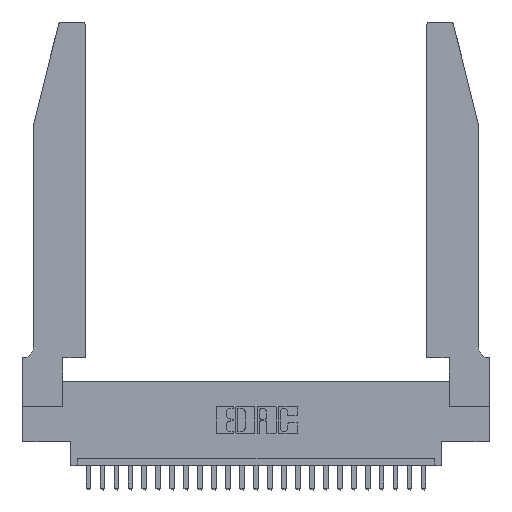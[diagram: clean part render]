
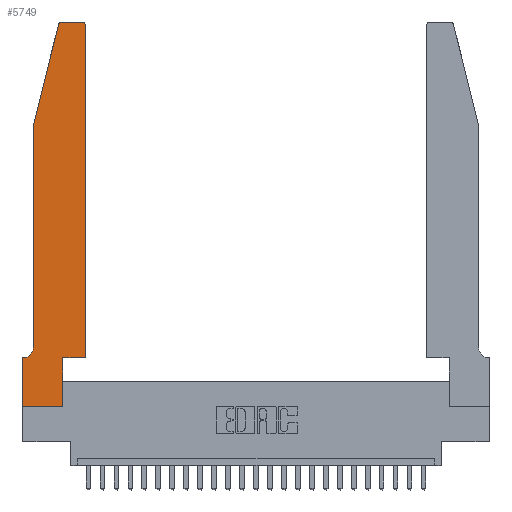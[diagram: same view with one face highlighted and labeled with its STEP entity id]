
A CAD part, top view. The second image highlights one B-rep face of the part: STEP entity #5749.
In plain terms, the highlighted planar face has unit normal (0, 0, 1).
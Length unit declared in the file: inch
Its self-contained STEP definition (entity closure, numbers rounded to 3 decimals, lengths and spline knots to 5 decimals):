
#238 = ORIENTED_EDGE ( 'NONE', *, *, #6319, .T. ) ;
#380 = DIRECTION ( 'NONE',  ( 1., 0., 0. ) ) ;
#554 = AXIS2_PLACEMENT_3D ( 'NONE', #16394, #8370, #4819 ) ;
#911 = VERTEX_POINT ( 'NONE', #15841 ) ;
#964 = DIRECTION ( 'NONE',  ( 1., 0., 0. ) ) ;
#1431 = EDGE_CURVE ( 'NONE', #16127, #13014, #11817, .T. ) ;
#2209 = LINE ( 'NONE', #9297, #5971 ) ;
#2292 = LINE ( 'NONE', #18422, #3536 ) ;
#2298 = PLANE ( 'NONE',  #554 ) ;
#2306 = CARTESIAN_POINT ( 'NONE',  ( 0.25487, 2.72718, 0.37 ) ) ;
#2475 = LINE ( 'NONE', #12851, #16607 ) ;
#2971 = ORIENTED_EDGE ( 'NONE', *, *, #1431, .T. ) ;
#3141 = ORIENTED_EDGE ( 'NONE', *, *, #25940, .T. ) ;
#3298 = EDGE_CURVE ( 'NONE', #3597, #13988, #22091, .T. ) ;
#3417 = CARTESIAN_POINT ( 'NONE',  ( 0.284, 2.75, 0.37 ) ) ;
#3482 = VECTOR ( 'NONE', #380, 39.37008 ) ;
#3536 = VECTOR ( 'NONE', #10362, 39.37008 ) ;
#3597 = VERTEX_POINT ( 'NONE', #12074 ) ;
#3706 = VERTEX_POINT ( 'NONE', #9615 ) ;
#3900 = ORIENTED_EDGE ( 'NONE', *, *, #3298, .T. ) ;
#3927 = VECTOR ( 'NONE', #9488, 39.37008 ) ;
#4383 = CARTESIAN_POINT ( 'NONE',  ( 0.4505, 0.35, 0.37 ) ) ;
#4387 = AXIS2_PLACEMENT_3D ( 'NONE', #4671, #24674, #16696 ) ;
#4437 = VECTOR ( 'NONE', #12284, 39.37008 ) ;
#4560 = CARTESIAN_POINT ( 'NONE',  ( 0.4205, 2.75, 0.37 ) ) ;
#4671 = CARTESIAN_POINT ( 'NONE',  ( 0.284, 2.72, 0.37 ) ) ;
#4819 = DIRECTION ( 'NONE',  ( 1., 0., 0. ) ) ;
#5542 = ORIENTED_EDGE ( 'NONE', *, *, #9561, .T. ) ;
#5701 = CARTESIAN_POINT ( 'NONE',  ( 0.4205, 2.72, 0.37 ) ) ;
#5749 = ADVANCED_FACE ( 'NONE', ( #19429 ), #2298, .T. ) ;
#5970 = DIRECTION ( 'NONE',  ( 0., 0., -1. ) ) ;
#5971 = VECTOR ( 'NONE', #22456, 39.37008 ) ;
#5985 = ORIENTED_EDGE ( 'NONE', *, *, #17972, .T. ) ;
#6319 = EDGE_CURVE ( 'NONE', #911, #3597, #22878, .T. ) ;
#6457 = EDGE_CURVE ( 'NONE', #7160, #10774, #13100, .T. ) ;
#6621 = EDGE_CURVE ( 'NONE', #3706, #7160, #20052, .T. ) ;
#7160 = VERTEX_POINT ( 'NONE', #8840 ) ;
#7277 = CARTESIAN_POINT ( 'NONE',  ( 0.0755, 0.35, 0.37 ) ) ;
#7413 = EDGE_CURVE ( 'NONE', #10774, #14008, #25652, .T. ) ;
#8094 = VERTEX_POINT ( 'NONE', #3417 ) ;
#8370 = DIRECTION ( 'NONE',  ( 0., 0., 1. ) ) ;
#8683 = VECTOR ( 'NONE', #19162, 39.37008 ) ;
#8840 = CARTESIAN_POINT ( 'NONE',  ( 0.0755, 0.42, 0.37 ) ) ;
#8891 = EDGE_CURVE ( 'NONE', #24763, #3706, #2292, .T. ) ;
#8940 = CIRCLE ( 'NONE', #4387, 0.03 ) ;
#9016 = VECTOR ( 'NONE', #964, 39.37008 ) ;
#9297 = CARTESIAN_POINT ( 'NONE',  ( 0., 0., 0.37 ) ) ;
#9488 = DIRECTION ( 'NONE',  ( 0., 1., 0. ) ) ;
#9561 = EDGE_CURVE ( 'NONE', #14008, #911, #2209, .T. ) ;
#9615 = CARTESIAN_POINT ( 'NONE',  ( 0.0755, 2., 0.37 ) ) ;
#9693 = VERTEX_POINT ( 'NONE', #4383 ) ;
#9786 = DIRECTION ( 'NONE',  ( 0., 0., 1. ) ) ;
#10362 = DIRECTION ( 'NONE',  ( -0.239, -0.971, 0. ) ) ;
#10774 = VERTEX_POINT ( 'NONE', #13089 ) ;
#10858 = EDGE_LOOP ( 'NONE', ( #12566, #3141, #24924, #20166, #24856, #14126, #5542, #238, #3900, #5985, #14589, #2971 ) ) ;
#11789 = DIRECTION ( 'NONE',  ( 1., 0., 0. ) ) ;
#11817 = CIRCLE ( 'NONE', #20412, 0.03 ) ;
#11958 = CARTESIAN_POINT ( 'NONE',  ( 0.0055, 0.42, 0.37 ) ) ;
#12074 = CARTESIAN_POINT ( 'NONE',  ( 0.2865, 0., 0.37 ) ) ;
#12284 = DIRECTION ( 'NONE',  ( 0., 1., 0. ) ) ;
#12566 = ORIENTED_EDGE ( 'NONE', *, *, #16043, .T. ) ;
#12734 = CARTESIAN_POINT ( 'NONE',  ( 0.2865, 0.35, 0.37 ) ) ;
#12851 = CARTESIAN_POINT ( 'NONE',  ( 0.2605, 2.75, 0.37 ) ) ;
#13014 = VERTEX_POINT ( 'NONE', #4560 ) ;
#13089 = CARTESIAN_POINT ( 'NONE',  ( 0.0055, 0.35, 0.37 ) ) ;
#13100 = CIRCLE ( 'NONE', #17651, 0.07 ) ;
#13799 = CARTESIAN_POINT ( 'NONE',  ( 0.4505, 0.35, 0.37 ) ) ;
#13988 = VERTEX_POINT ( 'NONE', #12734 ) ;
#14008 = VERTEX_POINT ( 'NONE', #22835 ) ;
#14126 = ORIENTED_EDGE ( 'NONE', *, *, #7413, .T. ) ;
#14589 = ORIENTED_EDGE ( 'NONE', *, *, #21708, .T. ) ;
#15290 = LINE ( 'NONE', #18166, #3927 ) ;
#15841 = CARTESIAN_POINT ( 'NONE',  ( 0., 0., 0.37 ) ) ;
#16043 = EDGE_CURVE ( 'NONE', #13014, #8094, #2475, .T. ) ;
#16127 = VERTEX_POINT ( 'NONE', #21008 ) ;
#16394 = CARTESIAN_POINT ( 'NONE',  ( 0., 0.35, 0.37 ) ) ;
#16607 = VECTOR ( 'NONE', #23128, 39.37008 ) ;
#16696 = DIRECTION ( 'NONE',  ( 1., 0., 0. ) ) ;
#17217 = CARTESIAN_POINT ( 'NONE',  ( 0., 0., 0.37 ) ) ;
#17651 = AXIS2_PLACEMENT_3D ( 'NONE', #11958, #5970, #20070 ) ;
#17972 = EDGE_CURVE ( 'NONE', #13988, #9693, #23040, .T. ) ;
#18166 = CARTESIAN_POINT ( 'NONE',  ( 0.4505, 0.35, 0.37 ) ) ;
#18422 = CARTESIAN_POINT ( 'NONE',  ( 0.0755, 2., 0.37 ) ) ;
#19091 = VECTOR ( 'NONE', #19621, 39.37008 ) ;
#19162 = DIRECTION ( 'NONE',  ( 0., -1., 0. ) ) ;
#19429 = FACE_OUTER_BOUND ( 'NONE', #10858, .T. ) ;
#19621 = DIRECTION ( 'NONE',  ( -1., 0., 0. ) ) ;
#20052 = LINE ( 'NONE', #25203, #8683 ) ;
#20070 = DIRECTION ( 'NONE',  ( -1., 0., 0. ) ) ;
#20166 = ORIENTED_EDGE ( 'NONE', *, *, #6621, .T. ) ;
#20412 = AXIS2_PLACEMENT_3D ( 'NONE', #5701, #9786, #11789 ) ;
#21008 = CARTESIAN_POINT ( 'NONE',  ( 0.4505, 2.72, 0.37 ) ) ;
#21708 = EDGE_CURVE ( 'NONE', #9693, #16127, #15290, .T. ) ;
#22091 = LINE ( 'NONE', #23900, #4437 ) ;
#22456 = DIRECTION ( 'NONE',  ( 0., -1., 0. ) ) ;
#22835 = CARTESIAN_POINT ( 'NONE',  ( 0., 0.35, 0.37 ) ) ;
#22878 = LINE ( 'NONE', #17217, #9016 ) ;
#23040 = LINE ( 'NONE', #13799, #3482 ) ;
#23128 = DIRECTION ( 'NONE',  ( -1., 0., 0. ) ) ;
#23900 = CARTESIAN_POINT ( 'NONE',  ( 0.2865, 0.35, 0.37 ) ) ;
#24674 = DIRECTION ( 'NONE',  ( 0., 0., 1. ) ) ;
#24763 = VERTEX_POINT ( 'NONE', #2306 ) ;
#24856 = ORIENTED_EDGE ( 'NONE', *, *, #6457, .T. ) ;
#24924 = ORIENTED_EDGE ( 'NONE', *, *, #8891, .T. ) ;
#25203 = CARTESIAN_POINT ( 'NONE',  ( 0.0755, 2., 0.37 ) ) ;
#25652 = LINE ( 'NONE', #7277, #19091 ) ;
#25940 = EDGE_CURVE ( 'NONE', #8094, #24763, #8940, .T. ) ;
